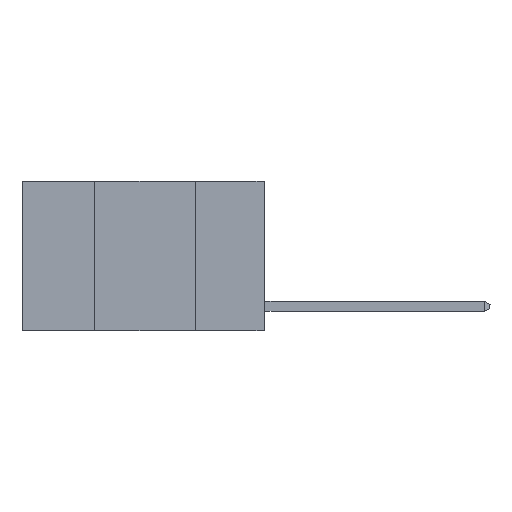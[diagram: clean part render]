
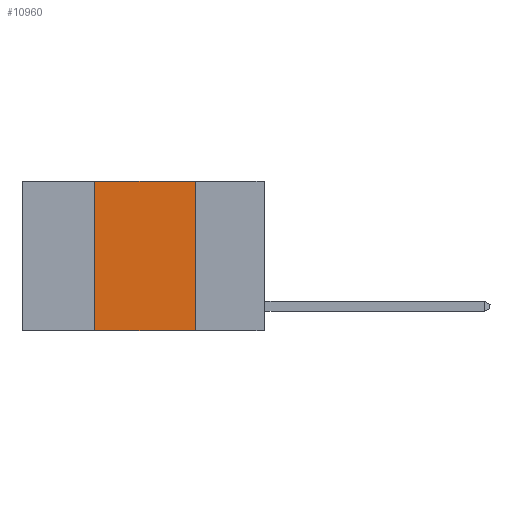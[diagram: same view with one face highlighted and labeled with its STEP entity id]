
A CAD part, left-side view. The second image highlights one B-rep face of the part: STEP entity #10960.
In plain terms, the highlighted planar face has unit normal (-1, 0, 0).
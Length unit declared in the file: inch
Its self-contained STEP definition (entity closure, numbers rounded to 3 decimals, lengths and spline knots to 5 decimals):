
#893 = EDGE_CURVE ( 'NONE', #20244, #19132, #10869, .T. ) ;
#1006 = CARTESIAN_POINT ( 'NONE',  ( 0., 0.42, 0. ) ) ;
#1130 = EDGE_CURVE ( 'NONE', #4007, #11633, #4858, .T. ) ;
#2647 = CARTESIAN_POINT ( 'NONE',  ( 0., 0.17, 0. ) ) ;
#4007 = VERTEX_POINT ( 'NONE', #9491 ) ;
#4474 = ORIENTED_EDGE ( 'NONE', *, *, #12853, .F. ) ;
#4600 = CARTESIAN_POINT ( 'NONE',  ( 0., 0.17, -0.37 ) ) ;
#4858 = LINE ( 'NONE', #12600, #13624 ) ;
#5067 = CARTESIAN_POINT ( 'NONE',  ( 0., 0.42, 0. ) ) ;
#5341 = AXIS2_PLACEMENT_3D ( 'NONE', #12965, #9528, #21449 ) ;
#5457 = FACE_OUTER_BOUND ( 'NONE', #19227, .T. ) ;
#6832 = DIRECTION ( 'NONE',  ( 0., 0., 1. ) ) ;
#8319 = CARTESIAN_POINT ( 'NONE',  ( 0., 0.17, 0. ) ) ;
#8911 = ORIENTED_EDGE ( 'NONE', *, *, #1130, .T. ) ;
#9491 = CARTESIAN_POINT ( 'NONE',  ( 0., 0.42, -0.37 ) ) ;
#9528 = DIRECTION ( 'NONE',  ( 1., 0., 0. ) ) ;
#10263 = LINE ( 'NONE', #5067, #18830 ) ;
#10786 = ORIENTED_EDGE ( 'NONE', *, *, #893, .F. ) ;
#10869 = LINE ( 'NONE', #11542, #14423 ) ;
#10960 = ADVANCED_FACE ( 'NONE', ( #5457 ), #19782, .F. ) ;
#11306 = DIRECTION ( 'NONE',  ( 0., -1., 0. ) ) ;
#11331 = ORIENTED_EDGE ( 'NONE', *, *, #18529, .F. ) ;
#11522 = DIRECTION ( 'NONE',  ( 0., -1., 0. ) ) ;
#11542 = CARTESIAN_POINT ( 'NONE',  ( 0., 0.6, 0. ) ) ;
#11633 = VERTEX_POINT ( 'NONE', #4600 ) ;
#12172 = LINE ( 'NONE', #2647, #20692 ) ;
#12600 = CARTESIAN_POINT ( 'NONE',  ( 0., 0.6, -0.37 ) ) ;
#12853 = EDGE_CURVE ( 'NONE', #19132, #11633, #12172, .T. ) ;
#12965 = CARTESIAN_POINT ( 'NONE',  ( 0., 0.6, 0. ) ) ;
#13624 = VECTOR ( 'NONE', #11306, 39.37008 ) ;
#14423 = VECTOR ( 'NONE', #11522, 39.37008 ) ;
#18529 = EDGE_CURVE ( 'NONE', #4007, #20244, #10263, .T. ) ;
#18830 = VECTOR ( 'NONE', #6832, 39.37008 ) ;
#19132 = VERTEX_POINT ( 'NONE', #8319 ) ;
#19227 = EDGE_LOOP ( 'NONE', ( #4474, #10786, #11331, #8911 ) ) ;
#19782 = PLANE ( 'NONE',  #5341 ) ;
#19936 = DIRECTION ( 'NONE',  ( 0., 0., -1. ) ) ;
#20244 = VERTEX_POINT ( 'NONE', #1006 ) ;
#20692 = VECTOR ( 'NONE', #19936, 39.37008 ) ;
#21449 = DIRECTION ( 'NONE',  ( 0., 0., -1. ) ) ;
